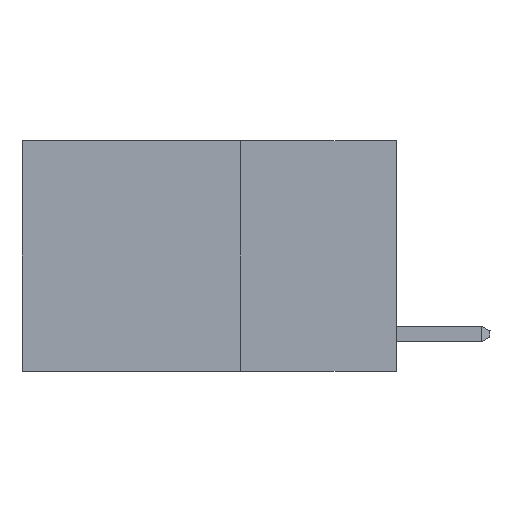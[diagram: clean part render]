
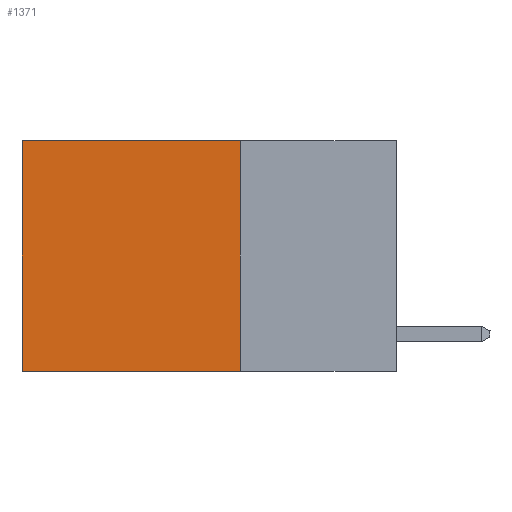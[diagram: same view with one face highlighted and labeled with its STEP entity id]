
A CAD part, left-side view. The second image highlights one B-rep face of the part: STEP entity #1371.
In plain terms, the highlighted planar face has unit normal (-1, 0, 0).
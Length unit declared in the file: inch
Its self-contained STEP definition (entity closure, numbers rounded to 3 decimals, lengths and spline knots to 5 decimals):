
#36 = CARTESIAN_POINT ( 'NONE',  ( 0.2625, 0.6, 0. ) ) ;
#242 = VERTEX_POINT ( 'NONE', #15039 ) ;
#590 = VECTOR ( 'NONE', #6627, 39.37008 ) ;
#819 = CARTESIAN_POINT ( 'NONE',  ( 0.2625, 0.6, -0.37 ) ) ;
#1037 = DIRECTION ( 'NONE',  ( 0., 1., 0. ) ) ;
#1371 = ADVANCED_FACE ( 'NONE', ( #9271 ), #15066, .F. ) ;
#2192 = EDGE_LOOP ( 'NONE', ( #14356, #5333, #14895, #13492 ) ) ;
#4064 = VECTOR ( 'NONE', #1037, 39.37008 ) ;
#4839 = CARTESIAN_POINT ( 'NONE',  ( 0.2625, 0.25, 0. ) ) ;
#5210 = DIRECTION ( 'NONE',  ( 0., 0., -1. ) ) ;
#5333 = ORIENTED_EDGE ( 'NONE', *, *, #9602, .F. ) ;
#5472 = AXIS2_PLACEMENT_3D ( 'NONE', #7035, #12362, #5695 ) ;
#5695 = DIRECTION ( 'NONE',  ( 0., 0., -1. ) ) ;
#5876 = LINE ( 'NONE', #4839, #4064 ) ;
#6627 = DIRECTION ( 'NONE',  ( 0., 1., 0. ) ) ;
#7035 = CARTESIAN_POINT ( 'NONE',  ( 0.2625, 0.25, 0. ) ) ;
#7184 = DIRECTION ( 'NONE',  ( 0., 0., -1. ) ) ;
#7429 = CARTESIAN_POINT ( 'NONE',  ( 0.2625, 0.25, 0. ) ) ;
#7958 = EDGE_CURVE ( 'NONE', #13244, #242, #11104, .T. ) ;
#8021 = VECTOR ( 'NONE', #7184, 39.37008 ) ;
#8254 = CARTESIAN_POINT ( 'NONE',  ( 0.2625, 0.6, 0. ) ) ;
#8771 = CARTESIAN_POINT ( 'NONE',  ( 0.2625, 0.25, 0. ) ) ;
#8996 = LINE ( 'NONE', #16008, #590 ) ;
#9102 = VERTEX_POINT ( 'NONE', #8254 ) ;
#9271 = FACE_OUTER_BOUND ( 'NONE', #2192, .T. ) ;
#9294 = VERTEX_POINT ( 'NONE', #819 ) ;
#9301 = EDGE_CURVE ( 'NONE', #13244, #9102, #5876, .T. ) ;
#9356 = VECTOR ( 'NONE', #5210, 39.37008 ) ;
#9602 = EDGE_CURVE ( 'NONE', #242, #9294, #8996, .T. ) ;
#11104 = LINE ( 'NONE', #8771, #8021 ) ;
#11671 = EDGE_CURVE ( 'NONE', #9102, #9294, #16397, .T. ) ;
#12362 = DIRECTION ( 'NONE',  ( 1., 0., 0. ) ) ;
#13244 = VERTEX_POINT ( 'NONE', #7429 ) ;
#13492 = ORIENTED_EDGE ( 'NONE', *, *, #9301, .T. ) ;
#14356 = ORIENTED_EDGE ( 'NONE', *, *, #11671, .T. ) ;
#14895 = ORIENTED_EDGE ( 'NONE', *, *, #7958, .F. ) ;
#15039 = CARTESIAN_POINT ( 'NONE',  ( 0.2625, 0.25, -0.37 ) ) ;
#15066 = PLANE ( 'NONE',  #5472 ) ;
#16008 = CARTESIAN_POINT ( 'NONE',  ( 0.2625, 0.25, -0.37 ) ) ;
#16397 = LINE ( 'NONE', #36, #9356 ) ;
